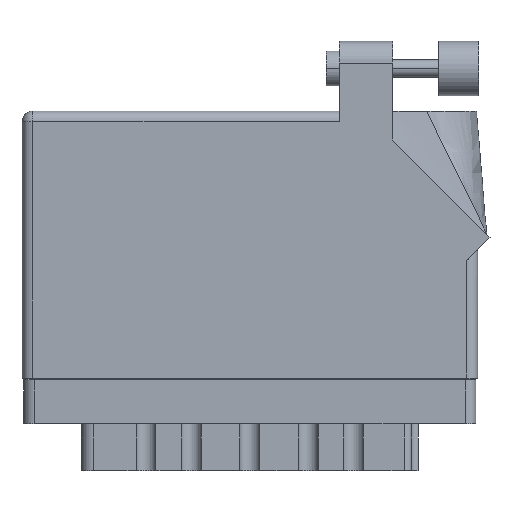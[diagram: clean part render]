
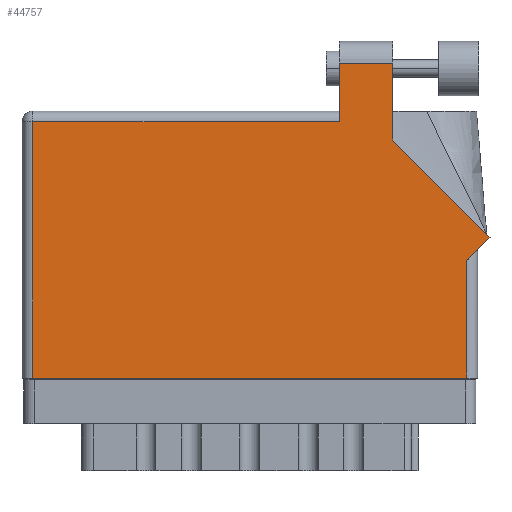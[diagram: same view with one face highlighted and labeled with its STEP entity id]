
A CAD part, front view. The second image highlights one B-rep face of the part: STEP entity #44757.
In plain terms, the highlighted face is planar.
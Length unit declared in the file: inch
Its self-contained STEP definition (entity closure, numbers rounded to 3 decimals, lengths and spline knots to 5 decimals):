
#1227 = CARTESIAN_POINT ( 'NONE',  ( 2.126, 1.36442, 0. ) ) ;
#1349 = VERTEX_POINT ( 'NONE', #36751 ) ;
#3156 = CARTESIAN_POINT ( 'NONE',  ( 1.819, 1.805, 0. ) ) ;
#3664 = EDGE_CURVE ( 'NONE', #1349, #13263, #27257, .T. ) ;
#3898 = EDGE_CURVE ( 'NONE', #11933, #7467, #23660, .T. ) ;
#4020 = VERTEX_POINT ( 'NONE', #3156 ) ;
#5336 = DIRECTION ( 'NONE',  ( 0., 0., -1. ) ) ;
#5527 = LINE ( 'NONE', #39302, #38406 ) ;
#5585 = EDGE_CURVE ( 'NONE', #25468, #25458, #45954, .T. ) ;
#6302 = VECTOR ( 'NONE', #11657, 39.37008 ) ;
#6946 = CARTESIAN_POINT ( 'NONE',  ( 0., 0., 0. ) ) ;
#7467 = VERTEX_POINT ( 'NONE', #12454 ) ;
#7515 = EDGE_CURVE ( 'NONE', #25458, #11933, #35513, .T. ) ;
#8157 = CARTESIAN_POINT ( 'NONE',  ( 2.55, 0.675, 0. ) ) ;
#8404 = VECTOR ( 'NONE', #41145, 39.37008 ) ;
#8685 = EDGE_CURVE ( 'NONE', #13821, #22898, #5527, .T. ) ;
#8746 = CARTESIAN_POINT ( 'NONE',  ( 2.55, 0.737, 0. ) ) ;
#9857 = DIRECTION ( 'NONE',  ( 0.707, 0.707, 0. ) ) ;
#9900 = EDGE_CURVE ( 'NONE', #22898, #4020, #45500, .T. ) ;
#11657 = DIRECTION ( 'NONE',  ( 0., -1., 0. ) ) ;
#11933 = VERTEX_POINT ( 'NONE', #8157 ) ;
#12244 = VECTOR ( 'NONE', #43203, 39.37008 ) ;
#12454 = CARTESIAN_POINT ( 'NONE',  ( 2.68271, 0.80771, 0. ) ) ;
#13263 = VERTEX_POINT ( 'NONE', #21192 ) ;
#13709 = VECTOR ( 'NONE', #46821, 39.37008 ) ;
#13821 = VERTEX_POINT ( 'NONE', #1227 ) ;
#13908 = ORIENTED_EDGE ( 'NONE', *, *, #30306, .T. ) ;
#14887 = CARTESIAN_POINT ( 'NONE',  ( 2.68271, 0.80771, 0. ) ) ;
#15990 = VECTOR ( 'NONE', #34315, 39.37008 ) ;
#16584 = CARTESIAN_POINT ( 'NONE',  ( 0.062, 0., 0. ) ) ;
#18269 = DIRECTION ( 'NONE',  ( -1., 0., 0. ) ) ;
#18468 = FACE_OUTER_BOUND ( 'NONE', #22835, .T. ) ;
#18781 = ORIENTED_EDGE ( 'NONE', *, *, #7515, .T. ) ;
#19191 = DIRECTION ( 'NONE',  ( -1., 0., 0. ) ) ;
#20671 = PLANE ( 'NONE',  #40233 ) ;
#21192 = CARTESIAN_POINT ( 'NONE',  ( 0.062, 1.468, 0. ) ) ;
#21804 = LINE ( 'NONE', #34520, #6302 ) ;
#22284 = CARTESIAN_POINT ( 'NONE',  ( 1.819, 1.805, 0. ) ) ;
#22724 = LINE ( 'NONE', #14887, #8404 ) ;
#22795 = CARTESIAN_POINT ( 'NONE',  ( 2.55, 0., 0. ) ) ;
#22835 = EDGE_LOOP ( 'NONE', ( #24215, #24158, #13908, #25978, #44123, #40361, #18781, #32592, #34452 ) ) ;
#22898 = VERTEX_POINT ( 'NONE', #35454 ) ;
#23660 = LINE ( 'NONE', #35741, #42847 ) ;
#24158 = ORIENTED_EDGE ( 'NONE', *, *, #9900, .T. ) ;
#24215 = ORIENTED_EDGE ( 'NONE', *, *, #8685, .T. ) ;
#24856 = CARTESIAN_POINT ( 'NONE',  ( 0., 1.53, 0. ) ) ;
#25458 = VERTEX_POINT ( 'NONE', #22795 ) ;
#25468 = VERTEX_POINT ( 'NONE', #16584 ) ;
#25978 = ORIENTED_EDGE ( 'NONE', *, *, #3664, .T. ) ;
#26326 = VECTOR ( 'NONE', #18269, 39.37008 ) ;
#27257 = LINE ( 'NONE', #34426, #41655 ) ;
#29219 = LINE ( 'NONE', #43301, #13709 ) ;
#30306 = EDGE_CURVE ( 'NONE', #4020, #1349, #29219, .T. ) ;
#31794 = DIRECTION ( 'NONE',  ( 0., 1., 0. ) ) ;
#32592 = ORIENTED_EDGE ( 'NONE', *, *, #3898, .T. ) ;
#32602 = EDGE_CURVE ( 'NONE', #13263, #25468, #21804, .T. ) ;
#34315 = DIRECTION ( 'NONE',  ( 1., 0., 0. ) ) ;
#34426 = CARTESIAN_POINT ( 'NONE',  ( 0., 1.468, 0. ) ) ;
#34452 = ORIENTED_EDGE ( 'NONE', *, *, #44277, .T. ) ;
#34520 = CARTESIAN_POINT ( 'NONE',  ( 0.062, 0., 0. ) ) ;
#35454 = CARTESIAN_POINT ( 'NONE',  ( 2.126, 1.805, 0. ) ) ;
#35513 = LINE ( 'NONE', #8746, #12244 ) ;
#35741 = CARTESIAN_POINT ( 'NONE',  ( 2.612, 0.737, 0. ) ) ;
#36751 = CARTESIAN_POINT ( 'NONE',  ( 1.819, 1.468, 0. ) ) ;
#38406 = VECTOR ( 'NONE', #31794, 39.37008 ) ;
#39302 = CARTESIAN_POINT ( 'NONE',  ( 2.126, 1.36442, 0. ) ) ;
#40233 = AXIS2_PLACEMENT_3D ( 'NONE', #24856, #5336, #43951 ) ;
#40361 = ORIENTED_EDGE ( 'NONE', *, *, #5585, .T. ) ;
#41145 = DIRECTION ( 'NONE',  ( -0.707, 0.707, 0. ) ) ;
#41655 = VECTOR ( 'NONE', #19191, 39.37008 ) ;
#42847 = VECTOR ( 'NONE', #9857, 39.37008 ) ;
#43203 = DIRECTION ( 'NONE',  ( 0., 1., 0. ) ) ;
#43301 = CARTESIAN_POINT ( 'NONE',  ( 1.819, 1.53, 0. ) ) ;
#43951 = DIRECTION ( 'NONE',  ( -1., 0., 0. ) ) ;
#44123 = ORIENTED_EDGE ( 'NONE', *, *, #32602, .T. ) ;
#44277 = EDGE_CURVE ( 'NONE', #7467, #13821, #22724, .T. ) ;
#44757 = ADVANCED_FACE ( 'NONE', ( #18468 ), #20671, .F. ) ;
#45500 = LINE ( 'NONE', #22284, #26326 ) ;
#45954 = LINE ( 'NONE', #6946, #15990 ) ;
#46821 = DIRECTION ( 'NONE',  ( 0., -1., 0. ) ) ;
